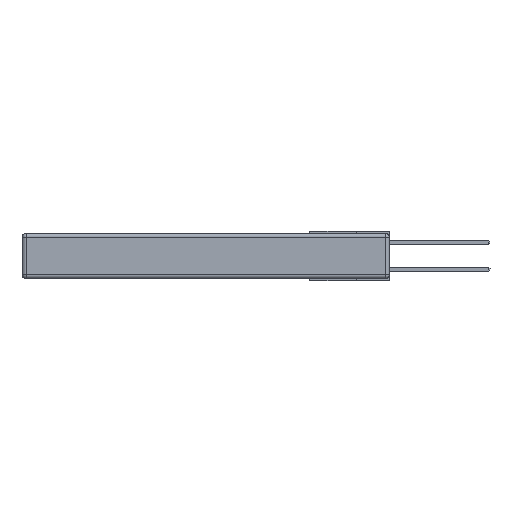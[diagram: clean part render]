
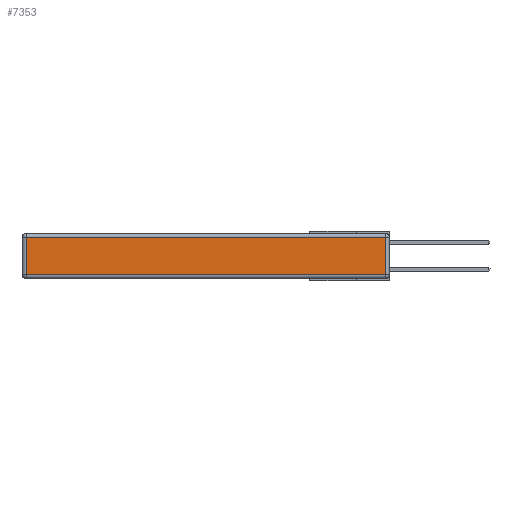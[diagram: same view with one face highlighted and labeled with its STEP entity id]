
A CAD part, left-side view. The second image highlights one B-rep face of the part: STEP entity #7353.
In plain terms, the highlighted planar face has unit normal (-1, 0, 0).
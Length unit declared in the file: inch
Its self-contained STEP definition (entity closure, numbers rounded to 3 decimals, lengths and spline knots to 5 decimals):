
#563 = DIRECTION ( 'NONE',  ( 0., 0., 1. ) ) ;
#661 = DIRECTION ( 'NONE',  ( 0., 1., 0. ) ) ;
#2232 = DIRECTION ( 'NONE',  ( 0., -1., 0. ) ) ;
#2429 = ORIENTED_EDGE ( 'NONE', *, *, #6314, .T. ) ;
#2705 = CARTESIAN_POINT ( 'NONE',  ( 0., 0.03, -0.343 ) ) ;
#2791 = EDGE_CURVE ( 'NONE', #26038, #12376, #13013, .T. ) ;
#4980 = LINE ( 'NONE', #27992, #27129 ) ;
#5340 = PLANE ( 'NONE',  #25674 ) ;
#5996 = EDGE_CURVE ( 'NONE', #12376, #30157, #4980, .T. ) ;
#6314 = EDGE_CURVE ( 'NONE', #18382, #26038, #8976, .T. ) ;
#7353 = ADVANCED_FACE ( 'NONE', ( #11874 ), #5340, .T. ) ;
#8976 = LINE ( 'NONE', #2705, #23020 ) ;
#9802 = LINE ( 'NONE', #16438, #17949 ) ;
#10482 = CARTESIAN_POINT ( 'NONE',  ( 0., 2.72, -0.03 ) ) ;
#10987 = CARTESIAN_POINT ( 'NONE',  ( 0., 0.03, -0.313 ) ) ;
#11874 = FACE_OUTER_BOUND ( 'NONE', #21762, .T. ) ;
#12376 = VERTEX_POINT ( 'NONE', #10482 ) ;
#12651 = DIRECTION ( 'NONE',  ( -1., 0., 0. ) ) ;
#12654 = CARTESIAN_POINT ( 'NONE',  ( 0., 2.75, -0.03 ) ) ;
#13013 = LINE ( 'NONE', #12654, #22598 ) ;
#15630 = CARTESIAN_POINT ( 'NONE',  ( 0., 0.03, -0.03 ) ) ;
#16438 = CARTESIAN_POINT ( 'NONE',  ( 0., 0., -0.313 ) ) ;
#17099 = DIRECTION ( 'NONE',  ( 0., 0., 1. ) ) ;
#17949 = VECTOR ( 'NONE', #2232, 39.37008 ) ;
#18382 = VERTEX_POINT ( 'NONE', #10987 ) ;
#19176 = EDGE_CURVE ( 'NONE', #30157, #18382, #9802, .T. ) ;
#21762 = EDGE_LOOP ( 'NONE', ( #23681, #2429, #30322, #23858 ) ) ;
#22598 = VECTOR ( 'NONE', #661, 39.37008 ) ;
#23020 = VECTOR ( 'NONE', #17099, 39.37008 ) ;
#23681 = ORIENTED_EDGE ( 'NONE', *, *, #19176, .T. ) ;
#23858 = ORIENTED_EDGE ( 'NONE', *, *, #5996, .T. ) ;
#24933 = CARTESIAN_POINT ( 'NONE',  ( 0., 2.72, -0.313 ) ) ;
#25674 = AXIS2_PLACEMENT_3D ( 'NONE', #28896, #12651, #563 ) ;
#26038 = VERTEX_POINT ( 'NONE', #15630 ) ;
#27129 = VECTOR ( 'NONE', #30386, 39.37008 ) ;
#27992 = CARTESIAN_POINT ( 'NONE',  ( 0., 2.72, -0.343 ) ) ;
#28896 = CARTESIAN_POINT ( 'NONE',  ( 0., 0., -0.343 ) ) ;
#30157 = VERTEX_POINT ( 'NONE', #24933 ) ;
#30322 = ORIENTED_EDGE ( 'NONE', *, *, #2791, .T. ) ;
#30386 = DIRECTION ( 'NONE',  ( 0., 0., -1. ) ) ;
